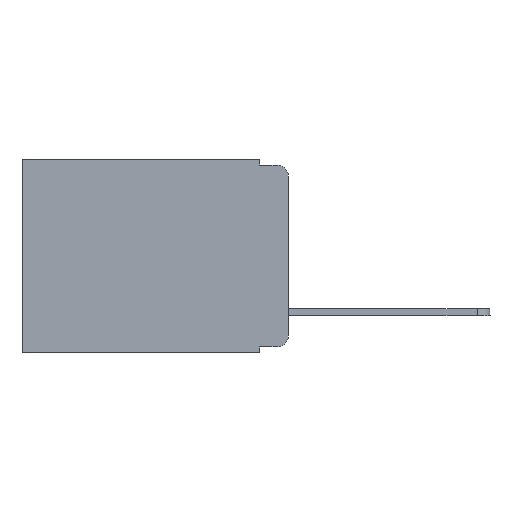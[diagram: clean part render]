
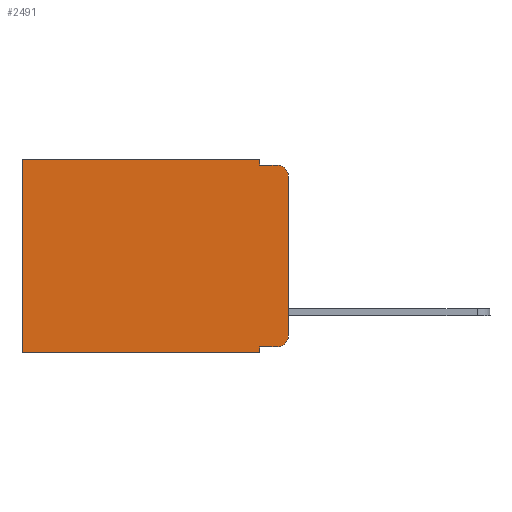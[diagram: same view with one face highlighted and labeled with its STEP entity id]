
A CAD part, left-side view. The second image highlights one B-rep face of the part: STEP entity #2491.
In plain terms, the highlighted planar face has unit normal (-1, 0, 0).
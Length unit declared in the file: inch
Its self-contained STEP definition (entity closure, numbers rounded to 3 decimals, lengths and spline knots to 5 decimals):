
#161 = ORIENTED_EDGE ( 'NONE', *, *, #1644, .T. ) ;
#283 = CARTESIAN_POINT ( 'NONE',  ( 0.298, 0.473, 0. ) ) ;
#350 = VECTOR ( 'NONE', #1275, 39.37008 ) ;
#401 = VERTEX_POINT ( 'NONE', #6531 ) ;
#447 = CARTESIAN_POINT ( 'NONE',  ( 0.298, 0.02, -0.333 ) ) ;
#449 = VECTOR ( 'NONE', #9525, 39.37008 ) ;
#632 = LINE ( 'NONE', #283, #6083 ) ;
#635 = EDGE_CURVE ( 'NONE', #7184, #4083, #5575, .T. ) ;
#654 = CARTESIAN_POINT ( 'NONE',  ( 0.298, 0.051, 0. ) ) ;
#720 = LINE ( 'NONE', #7690, #8812 ) ;
#934 = EDGE_LOOP ( 'NONE', ( #8371, #9485, #6647, #5008, #161, #5624, #2151, #8447, #3378, #2350 ) ) ;
#1275 = DIRECTION ( 'NONE',  ( 0., 1., 0. ) ) ;
#1602 = EDGE_CURVE ( 'NONE', #7184, #3955, #5920, .T. ) ;
#1644 = EDGE_CURVE ( 'NONE', #8404, #401, #4350, .T. ) ;
#2151 = ORIENTED_EDGE ( 'NONE', *, *, #7980, .F. ) ;
#2350 = ORIENTED_EDGE ( 'NONE', *, *, #4185, .T. ) ;
#2358 = VECTOR ( 'NONE', #6129, 39.37008 ) ;
#2488 = CARTESIAN_POINT ( 'NONE',  ( 0.298, 0.051, -0.01 ) ) ;
#2491 = ADVANCED_FACE ( 'NONE', ( #7955 ), #8525, .F. ) ;
#2529 = LINE ( 'NONE', #8751, #449 ) ;
#2638 = EDGE_CURVE ( 'NONE', #6492, #8875, #4683, .T. ) ;
#2654 = CARTESIAN_POINT ( 'NONE',  ( 0.298, 0.02, -0.01 ) ) ;
#3321 = CARTESIAN_POINT ( 'NONE',  ( 0.298, 0.051, -0.333 ) ) ;
#3378 = ORIENTED_EDGE ( 'NONE', *, *, #5350, .T. ) ;
#3438 = VECTOR ( 'NONE', #6217, 39.37008 ) ;
#3492 = CARTESIAN_POINT ( 'NONE',  ( 0.298, 0., -0.03 ) ) ;
#3955 = VERTEX_POINT ( 'NONE', #6216 ) ;
#3976 = CARTESIAN_POINT ( 'NONE',  ( 0.298, 0.051, -0.01 ) ) ;
#4083 = VERTEX_POINT ( 'NONE', #2654 ) ;
#4158 = LINE ( 'NONE', #3976, #3438 ) ;
#4185 = EDGE_CURVE ( 'NONE', #7828, #3955, #7074, .T. ) ;
#4200 = CARTESIAN_POINT ( 'NONE',  ( 0.298, 0.473, -0.343 ) ) ;
#4297 = CARTESIAN_POINT ( 'NONE',  ( 0.298, 0.051, -0.343 ) ) ;
#4350 = LINE ( 'NONE', #8205, #350 ) ;
#4545 = DIRECTION ( 'NONE',  ( -1., 0., 0. ) ) ;
#4683 = LINE ( 'NONE', #654, #9275 ) ;
#4715 = DIRECTION ( 'NONE',  ( 0., 1., 0. ) ) ;
#4911 = CARTESIAN_POINT ( 'NONE',  ( 0.298, 0.051, -0.333 ) ) ;
#5008 = ORIENTED_EDGE ( 'NONE', *, *, #8742, .F. ) ;
#5320 = CARTESIAN_POINT ( 'NONE',  ( 0.298, 0.051, 0. ) ) ;
#5350 = EDGE_CURVE ( 'NONE', #6492, #7828, #8520, .T. ) ;
#5377 = DIRECTION ( 'NONE',  ( -1., 0., 0. ) ) ;
#5488 = DIRECTION ( 'NONE',  ( 0., 0., -1. ) ) ;
#5505 = VERTEX_POINT ( 'NONE', #2488 ) ;
#5575 = CIRCLE ( 'NONE', #8469, 0.02 ) ;
#5624 = ORIENTED_EDGE ( 'NONE', *, *, #5827, .T. ) ;
#5637 = AXIS2_PLACEMENT_3D ( 'NONE', #9162, #5377, #6753 ) ;
#5804 = DIRECTION ( 'NONE',  ( 0., 0., -1. ) ) ;
#5827 = EDGE_CURVE ( 'NONE', #401, #8792, #632, .T. ) ;
#5920 = LINE ( 'NONE', #8871, #7745 ) ;
#6083 = VECTOR ( 'NONE', #8038, 39.37008 ) ;
#6097 = DIRECTION ( 'NONE',  ( 0., 0., -1. ) ) ;
#6129 = DIRECTION ( 'NONE',  ( 0., -1., 0. ) ) ;
#6172 = DIRECTION ( 'NONE',  ( 0., 0., -1. ) ) ;
#6216 = CARTESIAN_POINT ( 'NONE',  ( 0.298, 0., -0.313 ) ) ;
#6217 = DIRECTION ( 'NONE',  ( 0., -1., 0. ) ) ;
#6304 = EDGE_CURVE ( 'NONE', #5505, #4083, #4158, .T. ) ;
#6492 = VERTEX_POINT ( 'NONE', #4911 ) ;
#6531 = CARTESIAN_POINT ( 'NONE',  ( 0.298, 0.473, 0. ) ) ;
#6647 = ORIENTED_EDGE ( 'NONE', *, *, #6304, .F. ) ;
#6753 = DIRECTION ( 'NONE',  ( 0., 0., -1. ) ) ;
#7074 = CIRCLE ( 'NONE', #5637, 0.02 ) ;
#7184 = VERTEX_POINT ( 'NONE', #3492 ) ;
#7690 = CARTESIAN_POINT ( 'NONE',  ( 0.298, 0., -0.343 ) ) ;
#7745 = VECTOR ( 'NONE', #5804, 39.37008 ) ;
#7776 = AXIS2_PLACEMENT_3D ( 'NONE', #7786, #8560, #5488 ) ;
#7786 = CARTESIAN_POINT ( 'NONE',  ( 0.298, 0., 0. ) ) ;
#7828 = VERTEX_POINT ( 'NONE', #447 ) ;
#7955 = FACE_OUTER_BOUND ( 'NONE', #934, .T. ) ;
#7980 = EDGE_CURVE ( 'NONE', #8875, #8792, #720, .T. ) ;
#8038 = DIRECTION ( 'NONE',  ( 0., 0., -1. ) ) ;
#8205 = CARTESIAN_POINT ( 'NONE',  ( 0.298, 0., 0. ) ) ;
#8371 = ORIENTED_EDGE ( 'NONE', *, *, #1602, .F. ) ;
#8404 = VERTEX_POINT ( 'NONE', #5320 ) ;
#8408 = CARTESIAN_POINT ( 'NONE',  ( 0.298, 0.02, -0.03 ) ) ;
#8447 = ORIENTED_EDGE ( 'NONE', *, *, #2638, .F. ) ;
#8469 = AXIS2_PLACEMENT_3D ( 'NONE', #8408, #4545, #6097 ) ;
#8520 = LINE ( 'NONE', #3321, #2358 ) ;
#8525 = PLANE ( 'NONE',  #7776 ) ;
#8560 = DIRECTION ( 'NONE',  ( 1., 0., 0. ) ) ;
#8742 = EDGE_CURVE ( 'NONE', #8404, #5505, #2529, .T. ) ;
#8751 = CARTESIAN_POINT ( 'NONE',  ( 0.298, 0.051, 0. ) ) ;
#8792 = VERTEX_POINT ( 'NONE', #4200 ) ;
#8812 = VECTOR ( 'NONE', #4715, 39.37008 ) ;
#8871 = CARTESIAN_POINT ( 'NONE',  ( 0.298, 0., 0. ) ) ;
#8875 = VERTEX_POINT ( 'NONE', #4297 ) ;
#9162 = CARTESIAN_POINT ( 'NONE',  ( 0.298, 0.02, -0.313 ) ) ;
#9275 = VECTOR ( 'NONE', #6172, 39.37008 ) ;
#9485 = ORIENTED_EDGE ( 'NONE', *, *, #635, .T. ) ;
#9525 = DIRECTION ( 'NONE',  ( 0., 0., -1. ) ) ;
